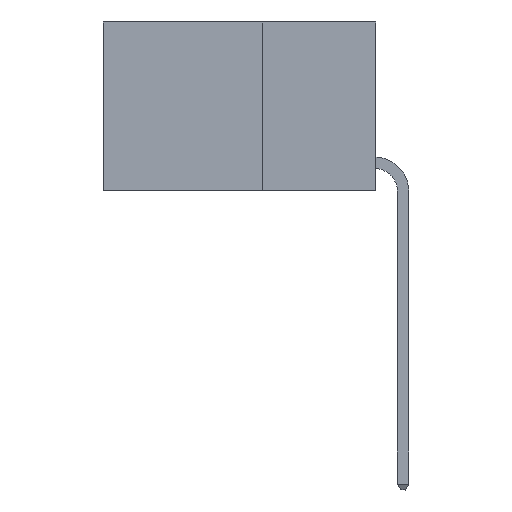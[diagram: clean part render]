
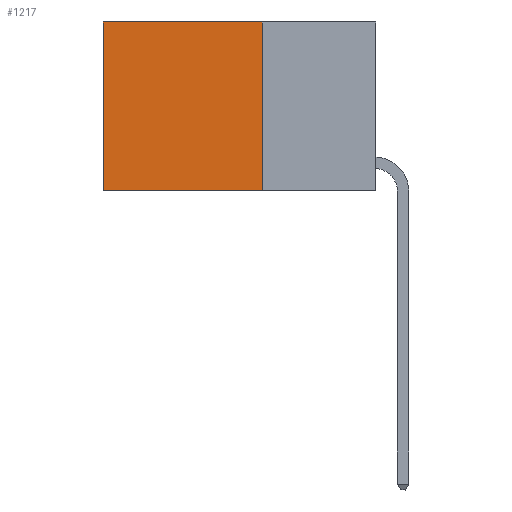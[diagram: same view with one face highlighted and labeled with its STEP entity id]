
A CAD part, left-side view. The second image highlights one B-rep face of the part: STEP entity #1217.
In plain terms, the highlighted planar face has unit normal (-1, 0, 0).
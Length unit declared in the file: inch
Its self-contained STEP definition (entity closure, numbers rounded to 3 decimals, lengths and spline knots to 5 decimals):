
#833 = ORIENTED_EDGE ( 'NONE', *, *, #15039, .T. ) ;
#1217 = ADVANCED_FACE ( 'NONE', ( #18865 ), #3726, .F. ) ;
#3022 = LINE ( 'NONE', #8234, #3733 ) ;
#3459 = VERTEX_POINT ( 'NONE', #28576 ) ;
#3726 = PLANE ( 'NONE',  #23109 ) ;
#3733 = VECTOR ( 'NONE', #23576, 39.37008 ) ;
#3887 = ORIENTED_EDGE ( 'NONE', *, *, #25438, .F. ) ;
#4017 = EDGE_CURVE ( 'NONE', #18719, #19748, #17091, .T. ) ;
#4870 = LINE ( 'NONE', #22678, #10846 ) ;
#8234 = CARTESIAN_POINT ( 'NONE',  ( 0.2625, 0.25, 0. ) ) ;
#8533 = DIRECTION ( 'NONE',  ( 1., 0., 0. ) ) ;
#9081 = DIRECTION ( 'NONE',  ( 0., 0., -1. ) ) ;
#10550 = EDGE_LOOP ( 'NONE', ( #22295, #28227, #3887, #833 ) ) ;
#10846 = VECTOR ( 'NONE', #11862, 39.37008 ) ;
#11862 = DIRECTION ( 'NONE',  ( 0., 0., -1. ) ) ;
#13172 = DIRECTION ( 'NONE',  ( 0., 1., 0. ) ) ;
#13576 = CARTESIAN_POINT ( 'NONE',  ( 0.2625, 0.25, 0. ) ) ;
#15039 = EDGE_CURVE ( 'NONE', #25675, #3459, #26616, .T. ) ;
#16341 = CARTESIAN_POINT ( 'NONE',  ( 0.2625, 0.25, 0. ) ) ;
#16670 = CARTESIAN_POINT ( 'NONE',  ( 0.2625, 0.25, 0. ) ) ;
#17091 = LINE ( 'NONE', #21773, #20744 ) ;
#18719 = VERTEX_POINT ( 'NONE', #27854 ) ;
#18865 = FACE_OUTER_BOUND ( 'NONE', #10550, .T. ) ;
#19748 = VERTEX_POINT ( 'NONE', #27436 ) ;
#20744 = VECTOR ( 'NONE', #13172, 39.37008 ) ;
#20962 = VECTOR ( 'NONE', #24930, 39.37008 ) ;
#21773 = CARTESIAN_POINT ( 'NONE',  ( 0.2625, 0.25, -0.37 ) ) ;
#22295 = ORIENTED_EDGE ( 'NONE', *, *, #24775, .T. ) ;
#22678 = CARTESIAN_POINT ( 'NONE',  ( 0.2625, 0.6, 0. ) ) ;
#23109 = AXIS2_PLACEMENT_3D ( 'NONE', #16670, #8533, #9081 ) ;
#23576 = DIRECTION ( 'NONE',  ( 0., 0., -1. ) ) ;
#24775 = EDGE_CURVE ( 'NONE', #3459, #19748, #4870, .T. ) ;
#24930 = DIRECTION ( 'NONE',  ( 0., 1., 0. ) ) ;
#25438 = EDGE_CURVE ( 'NONE', #25675, #18719, #3022, .T. ) ;
#25675 = VERTEX_POINT ( 'NONE', #13576 ) ;
#26616 = LINE ( 'NONE', #16341, #20962 ) ;
#27436 = CARTESIAN_POINT ( 'NONE',  ( 0.2625, 0.6, -0.37 ) ) ;
#27854 = CARTESIAN_POINT ( 'NONE',  ( 0.2625, 0.25, -0.37 ) ) ;
#28227 = ORIENTED_EDGE ( 'NONE', *, *, #4017, .F. ) ;
#28576 = CARTESIAN_POINT ( 'NONE',  ( 0.2625, 0.6, 0. ) ) ;
